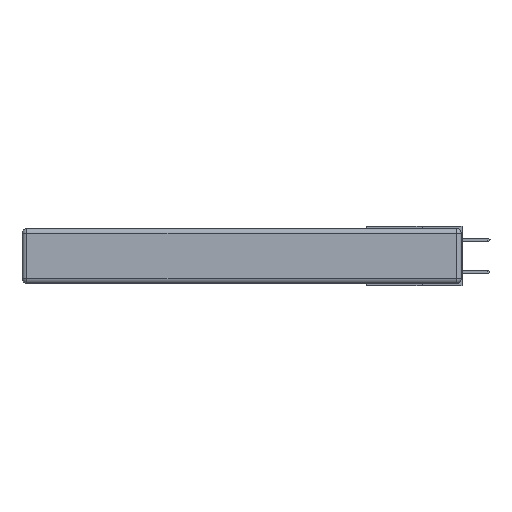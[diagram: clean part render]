
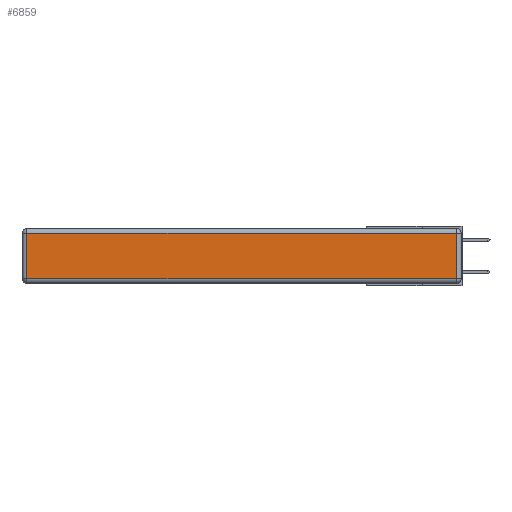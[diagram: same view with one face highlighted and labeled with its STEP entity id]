
A CAD part, left-side view. The second image highlights one B-rep face of the part: STEP entity #6859.
In plain terms, the highlighted planar face has unit normal (-1, 0, 0).
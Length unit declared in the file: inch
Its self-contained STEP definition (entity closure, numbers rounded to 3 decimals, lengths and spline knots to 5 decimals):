
#69 = CARTESIAN_POINT ( 'NONE',  ( 0., 2.72, -0.313 ) ) ;
#154 = CARTESIAN_POINT ( 'NONE',  ( 0., 0.03, -0.313 ) ) ;
#496 = VECTOR ( 'NONE', #8036, 39.37008 ) ;
#1191 = EDGE_CURVE ( 'NONE', #6758, #10518, #4225, .T. ) ;
#1511 = LINE ( 'NONE', #9682, #3932 ) ;
#1925 = EDGE_LOOP ( 'NONE', ( #15383, #10972, #8964, #3691 ) ) ;
#1943 = CARTESIAN_POINT ( 'NONE',  ( 0., 2.72, -0.03 ) ) ;
#2209 = AXIS2_PLACEMENT_3D ( 'NONE', #11239, #13441, #14572 ) ;
#2413 = DIRECTION ( 'NONE',  ( 0., 1., 0. ) ) ;
#3691 = ORIENTED_EDGE ( 'NONE', *, *, #14023, .T. ) ;
#3711 = CARTESIAN_POINT ( 'NONE',  ( 0., 2.75, -0.03 ) ) ;
#3804 = DIRECTION ( 'NONE',  ( 0., -1., 0. ) ) ;
#3932 = VECTOR ( 'NONE', #3804, 39.37008 ) ;
#4225 = LINE ( 'NONE', #13761, #496 ) ;
#4695 = VERTEX_POINT ( 'NONE', #1943 ) ;
#5142 = PLANE ( 'NONE',  #2209 ) ;
#5743 = DIRECTION ( 'NONE',  ( 0., 0., -1. ) ) ;
#6652 = VECTOR ( 'NONE', #5743, 39.37008 ) ;
#6758 = VERTEX_POINT ( 'NONE', #154 ) ;
#6859 = ADVANCED_FACE ( 'NONE', ( #11839 ), #5142, .T. ) ;
#8036 = DIRECTION ( 'NONE',  ( 0., 0., 1. ) ) ;
#8964 = ORIENTED_EDGE ( 'NONE', *, *, #15317, .T. ) ;
#9682 = CARTESIAN_POINT ( 'NONE',  ( 0., 0., -0.313 ) ) ;
#10330 = CARTESIAN_POINT ( 'NONE',  ( 0., 2.72, -0.343 ) ) ;
#10360 = LINE ( 'NONE', #3711, #12765 ) ;
#10518 = VERTEX_POINT ( 'NONE', #13137 ) ;
#10972 = ORIENTED_EDGE ( 'NONE', *, *, #1191, .T. ) ;
#11239 = CARTESIAN_POINT ( 'NONE',  ( 0., 0., -0.343 ) ) ;
#11455 = EDGE_CURVE ( 'NONE', #14870, #6758, #1511, .T. ) ;
#11839 = FACE_OUTER_BOUND ( 'NONE', #1925, .T. ) ;
#12765 = VECTOR ( 'NONE', #2413, 39.37008 ) ;
#13137 = CARTESIAN_POINT ( 'NONE',  ( 0., 0.03, -0.03 ) ) ;
#13441 = DIRECTION ( 'NONE',  ( -1., 0., 0. ) ) ;
#13761 = CARTESIAN_POINT ( 'NONE',  ( 0., 0.03, -0.343 ) ) ;
#13873 = LINE ( 'NONE', #10330, #6652 ) ;
#14023 = EDGE_CURVE ( 'NONE', #4695, #14870, #13873, .T. ) ;
#14572 = DIRECTION ( 'NONE',  ( 0., 0., 1. ) ) ;
#14870 = VERTEX_POINT ( 'NONE', #69 ) ;
#15317 = EDGE_CURVE ( 'NONE', #10518, #4695, #10360, .T. ) ;
#15383 = ORIENTED_EDGE ( 'NONE', *, *, #11455, .T. ) ;
